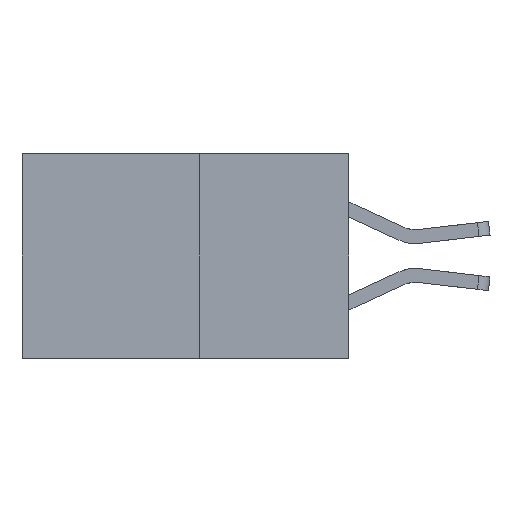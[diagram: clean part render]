
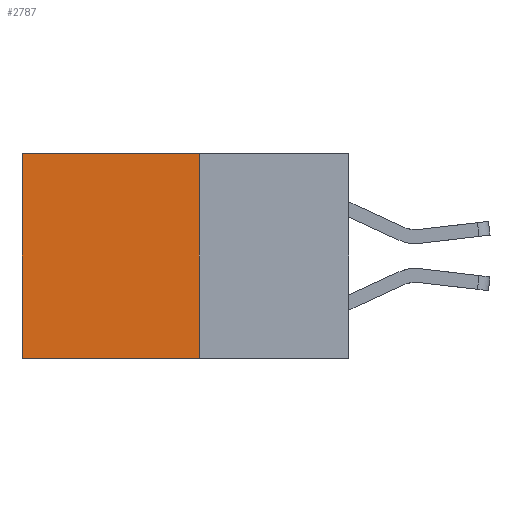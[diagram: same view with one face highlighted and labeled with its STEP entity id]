
A CAD part, left-side view. The second image highlights one B-rep face of the part: STEP entity #2787.
In plain terms, the highlighted planar face has unit normal (-1, 0, 0).
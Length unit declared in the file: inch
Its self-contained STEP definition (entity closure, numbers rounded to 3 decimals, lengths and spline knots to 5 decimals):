
#222 = DIRECTION ( 'NONE',  ( 0., 0., -1. ) ) ;
#250 = VERTEX_POINT ( 'NONE', #6401 ) ;
#438 = VECTOR ( 'NONE', #1758, 39.37008 ) ;
#652 = DIRECTION ( 'NONE',  ( 0., 1., 0. ) ) ;
#1319 = VERTEX_POINT ( 'NONE', #2320 ) ;
#1541 = EDGE_CURVE ( 'NONE', #250, #6184, #4404, .T. ) ;
#1758 = DIRECTION ( 'NONE',  ( 0., 0., -1. ) ) ;
#1875 = DIRECTION ( 'NONE',  ( 1., 0., 0. ) ) ;
#2221 = ORIENTED_EDGE ( 'NONE', *, *, #1541, .F. ) ;
#2320 = CARTESIAN_POINT ( 'NONE',  ( 0.277, 0.59, 0. ) ) ;
#2685 = LINE ( 'NONE', #6165, #5875 ) ;
#2689 = VECTOR ( 'NONE', #7449, 39.37008 ) ;
#2787 = ADVANCED_FACE ( 'NONE', ( #6836 ), #5639, .F. ) ;
#2846 = ORIENTED_EDGE ( 'NONE', *, *, #5076, .F. ) ;
#2969 = LINE ( 'NONE', #3654, #6158 ) ;
#3048 = DIRECTION ( 'NONE',  ( 0., 0., -1. ) ) ;
#3654 = CARTESIAN_POINT ( 'NONE',  ( 0.277, 0.59, -0.37 ) ) ;
#3778 = CARTESIAN_POINT ( 'NONE',  ( 0.277, 0.59, -0.37 ) ) ;
#4022 = CARTESIAN_POINT ( 'NONE',  ( 0.277, 0.27, 0. ) ) ;
#4328 = ORIENTED_EDGE ( 'NONE', *, *, #6675, .T. ) ;
#4404 = LINE ( 'NONE', #6542, #2689 ) ;
#4413 = CARTESIAN_POINT ( 'NONE',  ( 0.277, 0.27, -0.37 ) ) ;
#5076 = EDGE_CURVE ( 'NONE', #6794, #250, #7368, .T. ) ;
#5236 = EDGE_LOOP ( 'NONE', ( #4328, #2221, #2846, #5931 ) ) ;
#5639 = PLANE ( 'NONE',  #7366 ) ;
#5875 = VECTOR ( 'NONE', #652, 39.37008 ) ;
#5931 = ORIENTED_EDGE ( 'NONE', *, *, #6457, .T. ) ;
#6158 = VECTOR ( 'NONE', #222, 39.37008 ) ;
#6165 = CARTESIAN_POINT ( 'NONE',  ( 0.277, 0.27, 0. ) ) ;
#6184 = VERTEX_POINT ( 'NONE', #3778 ) ;
#6401 = CARTESIAN_POINT ( 'NONE',  ( 0.277, 0.27, -0.37 ) ) ;
#6457 = EDGE_CURVE ( 'NONE', #6794, #1319, #2685, .T. ) ;
#6542 = CARTESIAN_POINT ( 'NONE',  ( 0.277, 0.27, -0.37 ) ) ;
#6675 = EDGE_CURVE ( 'NONE', #1319, #6184, #2969, .T. ) ;
#6794 = VERTEX_POINT ( 'NONE', #4022 ) ;
#6836 = FACE_OUTER_BOUND ( 'NONE', #5236, .T. ) ;
#7366 = AXIS2_PLACEMENT_3D ( 'NONE', #7795, #1875, #3048 ) ;
#7368 = LINE ( 'NONE', #4413, #438 ) ;
#7449 = DIRECTION ( 'NONE',  ( 0., 1., 0. ) ) ;
#7795 = CARTESIAN_POINT ( 'NONE',  ( 0.277, 0.27, -0.37 ) ) ;
